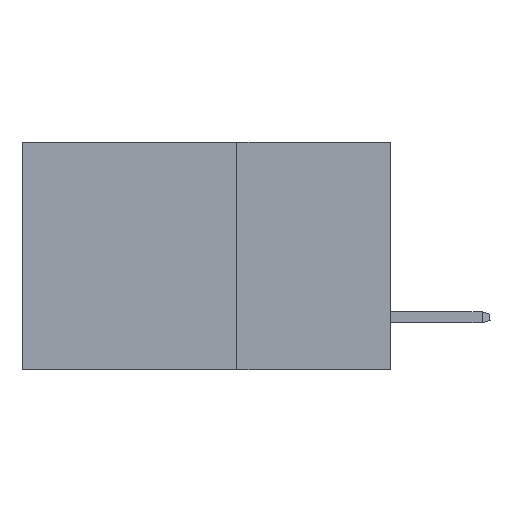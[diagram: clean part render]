
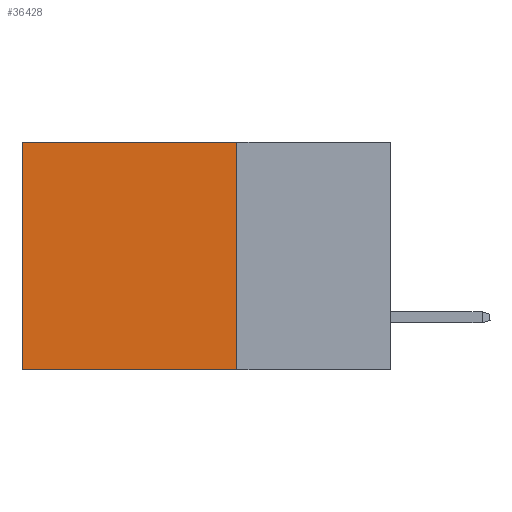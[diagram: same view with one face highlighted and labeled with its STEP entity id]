
A CAD part, left-side view. The second image highlights one B-rep face of the part: STEP entity #36428.
In plain terms, the highlighted planar face has unit normal (-1, 0, 0).
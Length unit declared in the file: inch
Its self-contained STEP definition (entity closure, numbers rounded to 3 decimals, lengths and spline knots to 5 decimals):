
#2340 = VERTEX_POINT ( 'NONE', #10830 ) ;
#4270 = LINE ( 'NONE', #8819, #22457 ) ;
#4521 = ORIENTED_EDGE ( 'NONE', *, *, #47128, .T. ) ;
#5843 = EDGE_CURVE ( 'NONE', #2340, #23593, #12482, .T. ) ;
#5986 = LINE ( 'NONE', #17330, #22462 ) ;
#6589 = VECTOR ( 'NONE', #15941, 39.37008 ) ;
#7690 = VERTEX_POINT ( 'NONE', #9632 ) ;
#7731 = CARTESIAN_POINT ( 'NONE',  ( 0.2875, 0.25, 0. ) ) ;
#8397 = VERTEX_POINT ( 'NONE', #41294 ) ;
#8819 = CARTESIAN_POINT ( 'NONE',  ( 0.2875, 0.25, 0. ) ) ;
#9632 = CARTESIAN_POINT ( 'NONE',  ( 0.2875, 0.6, -0.37 ) ) ;
#10830 = CARTESIAN_POINT ( 'NONE',  ( 0.2875, 0.25, 0. ) ) ;
#11969 = CARTESIAN_POINT ( 'NONE',  ( 0.2875, 0.25, -0.37 ) ) ;
#12482 = LINE ( 'NONE', #7731, #34642 ) ;
#15941 = DIRECTION ( 'NONE',  ( 0., 1., 0. ) ) ;
#16153 = EDGE_CURVE ( 'NONE', #8397, #7690, #20212, .T. ) ;
#16542 = CARTESIAN_POINT ( 'NONE',  ( 0.2875, 0.6, 0. ) ) ;
#17330 = CARTESIAN_POINT ( 'NONE',  ( 0.2875, 0.6, 0. ) ) ;
#19320 = DIRECTION ( 'NONE',  ( 0., 0., -1. ) ) ;
#19561 = DIRECTION ( 'NONE',  ( 0., 0., -1. ) ) ;
#20212 = LINE ( 'NONE', #11969, #6589 ) ;
#21732 = FACE_OUTER_BOUND ( 'NONE', #46881, .T. ) ;
#22457 = VECTOR ( 'NONE', #19320, 39.37008 ) ;
#22462 = VECTOR ( 'NONE', #42844, 39.37008 ) ;
#22731 = DIRECTION ( 'NONE',  ( 0., 1., 0. ) ) ;
#23530 = CARTESIAN_POINT ( 'NONE',  ( 0.2875, 0.25, 0. ) ) ;
#23593 = VERTEX_POINT ( 'NONE', #16542 ) ;
#27337 = ORIENTED_EDGE ( 'NONE', *, *, #41050, .F. ) ;
#27406 = ORIENTED_EDGE ( 'NONE', *, *, #5843, .T. ) ;
#29066 = AXIS2_PLACEMENT_3D ( 'NONE', #23530, #41884, #19561 ) ;
#34642 = VECTOR ( 'NONE', #22731, 39.37008 ) ;
#34713 = ORIENTED_EDGE ( 'NONE', *, *, #16153, .F. ) ;
#36428 = ADVANCED_FACE ( 'NONE', ( #21732 ), #45207, .F. ) ;
#41050 = EDGE_CURVE ( 'NONE', #2340, #8397, #4270, .T. ) ;
#41294 = CARTESIAN_POINT ( 'NONE',  ( 0.2875, 0.25, -0.37 ) ) ;
#41884 = DIRECTION ( 'NONE',  ( 1., 0., 0. ) ) ;
#42844 = DIRECTION ( 'NONE',  ( 0., 0., -1. ) ) ;
#45207 = PLANE ( 'NONE',  #29066 ) ;
#46881 = EDGE_LOOP ( 'NONE', ( #4521, #34713, #27337, #27406 ) ) ;
#47128 = EDGE_CURVE ( 'NONE', #23593, #7690, #5986, .T. ) ;
